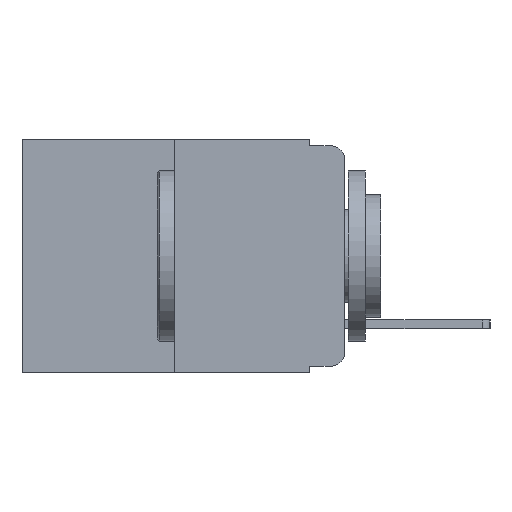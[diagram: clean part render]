
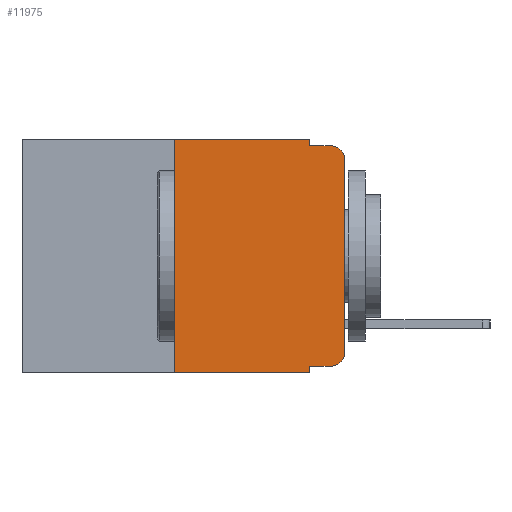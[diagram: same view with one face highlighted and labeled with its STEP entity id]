
A CAD part, left-side view. The second image highlights one B-rep face of the part: STEP entity #11975.
In plain terms, the highlighted planar face has unit normal (-1, 0, 0).
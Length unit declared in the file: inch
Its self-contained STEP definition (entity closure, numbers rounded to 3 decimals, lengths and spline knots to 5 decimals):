
#23 = DIRECTION ( 'NONE',  ( 0., 0., 1. ) ) ;
#219 = CARTESIAN_POINT ( 'NONE',  ( 0., 0.473, -0.343 ) ) ;
#224 = ORIENTED_EDGE ( 'NONE', *, *, #23169, .T. ) ;
#778 = EDGE_CURVE ( 'NONE', #12436, #7587, #7946, .T. ) ;
#1165 = CARTESIAN_POINT ( 'NONE',  ( 0., 0.051, -0.01 ) ) ;
#1876 = CARTESIAN_POINT ( 'NONE',  ( 0., 0.25, 0. ) ) ;
#2031 = CIRCLE ( 'NONE', #2639, 0.02 ) ;
#2248 = LINE ( 'NONE', #10103, #11361 ) ;
#2464 = CARTESIAN_POINT ( 'NONE',  ( 0., 0.473, 0. ) ) ;
#2520 = EDGE_CURVE ( 'NONE', #14592, #5052, #10884, .T. ) ;
#2639 = AXIS2_PLACEMENT_3D ( 'NONE', #20474, #8987, #22405 ) ;
#2698 = CIRCLE ( 'NONE', #3643, 0.02 ) ;
#3103 = VECTOR ( 'NONE', #23, 39.37008 ) ;
#3643 = AXIS2_PLACEMENT_3D ( 'NONE', #6191, #19692, #8166 ) ;
#4009 = CARTESIAN_POINT ( 'NONE',  ( 0., 0., 0. ) ) ;
#4033 = DIRECTION ( 'NONE',  ( 0., -1., 0. ) ) ;
#4929 = DIRECTION ( 'NONE',  ( 0., 0., -1. ) ) ;
#5052 = VERTEX_POINT ( 'NONE', #6372 ) ;
#5147 = LINE ( 'NONE', #13673, #14824 ) ;
#5594 = ORIENTED_EDGE ( 'NONE', *, *, #6196, .T. ) ;
#5718 = VECTOR ( 'NONE', #21499, 39.37008 ) ;
#6191 = CARTESIAN_POINT ( 'NONE',  ( 0., 0.02, -0.03 ) ) ;
#6196 = EDGE_CURVE ( 'NONE', #12436, #8405, #13655, .T. ) ;
#6362 = PLANE ( 'NONE',  #14032 ) ;
#6372 = CARTESIAN_POINT ( 'NONE',  ( 0., 0.02, -0.01 ) ) ;
#6795 = ORIENTED_EDGE ( 'NONE', *, *, #16150, .F. ) ;
#7587 = VERTEX_POINT ( 'NONE', #1876 ) ;
#7737 = EDGE_CURVE ( 'NONE', #21738, #5052, #2698, .T. ) ;
#7946 = LINE ( 'NONE', #13001, #17581 ) ;
#8166 = DIRECTION ( 'NONE',  ( 0., 0., -1. ) ) ;
#8313 = ORIENTED_EDGE ( 'NONE', *, *, #12109, .F. ) ;
#8328 = DIRECTION ( 'NONE',  ( 1., 0., 0. ) ) ;
#8405 = VERTEX_POINT ( 'NONE', #12014 ) ;
#8614 = ORIENTED_EDGE ( 'NONE', *, *, #2520, .F. ) ;
#8987 = DIRECTION ( 'NONE',  ( -1., 0., 0. ) ) ;
#9151 = VECTOR ( 'NONE', #15864, 39.37008 ) ;
#9585 = VERTEX_POINT ( 'NONE', #23576 ) ;
#9715 = CARTESIAN_POINT ( 'NONE',  ( 0., 0., -0.313 ) ) ;
#10103 = CARTESIAN_POINT ( 'NONE',  ( 0., 0.473, 0. ) ) ;
#10158 = VERTEX_POINT ( 'NONE', #12018 ) ;
#10445 = ORIENTED_EDGE ( 'NONE', *, *, #778, .F. ) ;
#10884 = LINE ( 'NONE', #14192, #5718 ) ;
#10938 = VERTEX_POINT ( 'NONE', #10990 ) ;
#10990 = CARTESIAN_POINT ( 'NONE',  ( 0., 0.051, 0. ) ) ;
#11361 = VECTOR ( 'NONE', #15915, 39.37008 ) ;
#11580 = DIRECTION ( 'NONE',  ( 0., 0., 1. ) ) ;
#11590 = CARTESIAN_POINT ( 'NONE',  ( 0., 0.25, -0.343 ) ) ;
#11975 = ADVANCED_FACE ( 'NONE', ( #21168 ), #6362, .F. ) ;
#12014 = CARTESIAN_POINT ( 'NONE',  ( 0., 0.051, -0.343 ) ) ;
#12018 = CARTESIAN_POINT ( 'NONE',  ( 0., 0.02, -0.333 ) ) ;
#12109 = EDGE_CURVE ( 'NONE', #10938, #14592, #13060, .T. ) ;
#12112 = CARTESIAN_POINT ( 'NONE',  ( 0., 0.051, 0. ) ) ;
#12436 = VERTEX_POINT ( 'NONE', #11590 ) ;
#13001 = CARTESIAN_POINT ( 'NONE',  ( 0., 0.25, 0. ) ) ;
#13060 = LINE ( 'NONE', #16514, #18157 ) ;
#13104 = ORIENTED_EDGE ( 'NONE', *, *, #7737, .T. ) ;
#13609 = VERTEX_POINT ( 'NONE', #9715 ) ;
#13655 = LINE ( 'NONE', #219, #9151 ) ;
#13673 = CARTESIAN_POINT ( 'NONE',  ( 0., 0.051, -0.333 ) ) ;
#14032 = AXIS2_PLACEMENT_3D ( 'NONE', #2464, #8328, #21789 ) ;
#14113 = EDGE_LOOP ( 'NONE', ( #224, #13104, #8614, #8313, #6795, #10445, #5594, #23929, #19226, #21938 ) ) ;
#14192 = CARTESIAN_POINT ( 'NONE',  ( 0., 0.051, -0.01 ) ) ;
#14383 = EDGE_CURVE ( 'NONE', #9585, #8405, #20729, .T. ) ;
#14592 = VERTEX_POINT ( 'NONE', #1165 ) ;
#14824 = VECTOR ( 'NONE', #4033, 39.37008 ) ;
#15643 = VECTOR ( 'NONE', #21766, 39.37008 ) ;
#15864 = DIRECTION ( 'NONE',  ( 0., -1., 0. ) ) ;
#15915 = DIRECTION ( 'NONE',  ( 0., -1., 0. ) ) ;
#16150 = EDGE_CURVE ( 'NONE', #7587, #10938, #2248, .T. ) ;
#16313 = CARTESIAN_POINT ( 'NONE',  ( 0., 0., -0.03 ) ) ;
#16514 = CARTESIAN_POINT ( 'NONE',  ( 0., 0.051, 0. ) ) ;
#17581 = VECTOR ( 'NONE', #11580, 39.37008 ) ;
#18157 = VECTOR ( 'NONE', #4929, 39.37008 ) ;
#18505 = LINE ( 'NONE', #4009, #3103 ) ;
#19226 = ORIENTED_EDGE ( 'NONE', *, *, #25036, .T. ) ;
#19692 = DIRECTION ( 'NONE',  ( -1., 0., 0. ) ) ;
#19976 = EDGE_CURVE ( 'NONE', #10158, #13609, #2031, .T. ) ;
#20474 = CARTESIAN_POINT ( 'NONE',  ( 0., 0.02, -0.313 ) ) ;
#20729 = LINE ( 'NONE', #12112, #15643 ) ;
#21168 = FACE_OUTER_BOUND ( 'NONE', #14113, .T. ) ;
#21499 = DIRECTION ( 'NONE',  ( 0., -1., 0. ) ) ;
#21738 = VERTEX_POINT ( 'NONE', #16313 ) ;
#21766 = DIRECTION ( 'NONE',  ( 0., 0., -1. ) ) ;
#21789 = DIRECTION ( 'NONE',  ( 0., 0., -1. ) ) ;
#21938 = ORIENTED_EDGE ( 'NONE', *, *, #19976, .T. ) ;
#22405 = DIRECTION ( 'NONE',  ( 0., 0., -1. ) ) ;
#23169 = EDGE_CURVE ( 'NONE', #13609, #21738, #18505, .T. ) ;
#23576 = CARTESIAN_POINT ( 'NONE',  ( 0., 0.051, -0.333 ) ) ;
#23929 = ORIENTED_EDGE ( 'NONE', *, *, #14383, .F. ) ;
#25036 = EDGE_CURVE ( 'NONE', #9585, #10158, #5147, .T. ) ;
